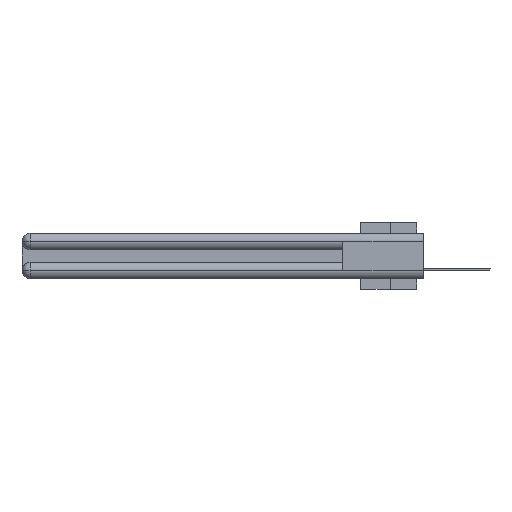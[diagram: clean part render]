
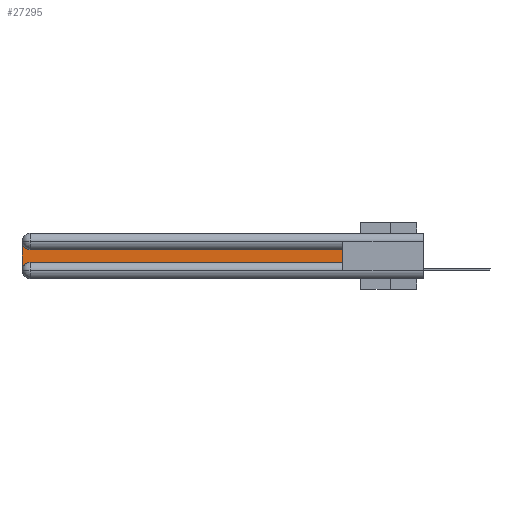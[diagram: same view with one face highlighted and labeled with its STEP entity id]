
A CAD part, left-side view. The second image highlights one B-rep face of the part: STEP entity #27295.
In plain terms, the highlighted planar face has unit normal (-1, 0, 0).
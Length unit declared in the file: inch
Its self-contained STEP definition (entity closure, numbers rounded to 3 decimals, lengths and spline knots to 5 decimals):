
#721 = EDGE_CURVE ( 'NONE', #13589, #35655, #24511, .T. ) ;
#1284 = ORIENTED_EDGE ( 'NONE', *, *, #33285, .T. ) ;
#1343 = LINE ( 'NONE', #18282, #25148 ) ;
#2421 = EDGE_CURVE ( 'NONE', #35655, #9357, #7483, .T. ) ;
#2525 = EDGE_LOOP ( 'NONE', ( #8137, #1284, #23221, #5854, #29954, #27167 ) ) ;
#3561 = EDGE_CURVE ( 'NONE', #22758, #7211, #1343, .T. ) ;
#4116 = CARTESIAN_POINT ( 'NONE',  ( 0.075, 3., -0.1225 ) ) ;
#5854 = ORIENTED_EDGE ( 'NONE', *, *, #2421, .T. ) ;
#7211 = VERTEX_POINT ( 'NONE', #9144 ) ;
#7413 = CARTESIAN_POINT ( 'NONE',  ( 0.075, 0.6, -0.2175 ) ) ;
#7483 = CIRCLE ( 'NONE', #28123, 0.06 ) ;
#7709 = CARTESIAN_POINT ( 'NONE',  ( 0.075, 3., -0.2175 ) ) ;
#8137 = ORIENTED_EDGE ( 'NONE', *, *, #3561, .T. ) ;
#9144 = CARTESIAN_POINT ( 'NONE',  ( 0.075, 2.94, -0.1225 ) ) ;
#9357 = VERTEX_POINT ( 'NONE', #12014 ) ;
#9602 = AXIS2_PLACEMENT_3D ( 'NONE', #32235, #18549, #21319 ) ;
#9610 = DIRECTION ( 'NONE',  ( 0., 1., 0. ) ) ;
#10001 = CARTESIAN_POINT ( 'NONE',  ( 0.075, 3., -0.0625 ) ) ;
#12014 = CARTESIAN_POINT ( 'NONE',  ( 0.075, 2.94, -0.2175 ) ) ;
#12830 = AXIS2_PLACEMENT_3D ( 'NONE', #4116, #15349, #26619 ) ;
#13589 = VERTEX_POINT ( 'NONE', #10001 ) ;
#15349 = DIRECTION ( 'NONE',  ( 1., 0., 0. ) ) ;
#16695 = VERTEX_POINT ( 'NONE', #34520 ) ;
#17728 = EDGE_CURVE ( 'NONE', #9357, #16695, #32716, .T. ) ;
#18282 = CARTESIAN_POINT ( 'NONE',  ( 0.075, 0.6, -0.1225 ) ) ;
#18447 = CIRCLE ( 'NONE', #9602, 0.06 ) ;
#18542 = LINE ( 'NONE', #29819, #27892 ) ;
#18549 = DIRECTION ( 'NONE',  ( 1., 0., 0. ) ) ;
#18788 = VECTOR ( 'NONE', #35772, 39.37008 ) ;
#20884 = FACE_OUTER_BOUND ( 'NONE', #2525, .T. ) ;
#21319 = DIRECTION ( 'NONE',  ( 0., 0., -1. ) ) ;
#21801 = VECTOR ( 'NONE', #35845, 39.37008 ) ;
#22758 = VERTEX_POINT ( 'NONE', #27921 ) ;
#23209 = CARTESIAN_POINT ( 'NONE',  ( 0.075, 3., -0.2775 ) ) ;
#23221 = ORIENTED_EDGE ( 'NONE', *, *, #721, .T. ) ;
#24361 = DIRECTION ( 'NONE',  ( 0., 0., -1. ) ) ;
#24511 = LINE ( 'NONE', #7709, #18788 ) ;
#25148 = VECTOR ( 'NONE', #9610, 39.37008 ) ;
#26619 = DIRECTION ( 'NONE',  ( 0., 0., -1. ) ) ;
#27167 = ORIENTED_EDGE ( 'NONE', *, *, #32152, .T. ) ;
#27295 = ADVANCED_FACE ( 'NONE', ( #20884 ), #35110, .F. ) ;
#27892 = VECTOR ( 'NONE', #33327, 39.37008 ) ;
#27921 = CARTESIAN_POINT ( 'NONE',  ( 0.075, 0.6, -0.1225 ) ) ;
#28123 = AXIS2_PLACEMENT_3D ( 'NONE', #32508, #35618, #24361 ) ;
#29819 = CARTESIAN_POINT ( 'NONE',  ( 0.075, 0.6, -0.2175 ) ) ;
#29954 = ORIENTED_EDGE ( 'NONE', *, *, #17728, .T. ) ;
#32152 = EDGE_CURVE ( 'NONE', #16695, #22758, #18542, .T. ) ;
#32235 = CARTESIAN_POINT ( 'NONE',  ( 0.075, 2.94, -0.0625 ) ) ;
#32508 = CARTESIAN_POINT ( 'NONE',  ( 0.075, 2.94, -0.2775 ) ) ;
#32716 = LINE ( 'NONE', #7413, #21801 ) ;
#33285 = EDGE_CURVE ( 'NONE', #7211, #13589, #18447, .T. ) ;
#33327 = DIRECTION ( 'NONE',  ( 0., 0., 1. ) ) ;
#34520 = CARTESIAN_POINT ( 'NONE',  ( 0.075, 0.6, -0.2175 ) ) ;
#35110 = PLANE ( 'NONE',  #12830 ) ;
#35618 = DIRECTION ( 'NONE',  ( 1., 0., 0. ) ) ;
#35655 = VERTEX_POINT ( 'NONE', #23209 ) ;
#35772 = DIRECTION ( 'NONE',  ( 0., 0., -1. ) ) ;
#35845 = DIRECTION ( 'NONE',  ( 0., -1., 0. ) ) ;
